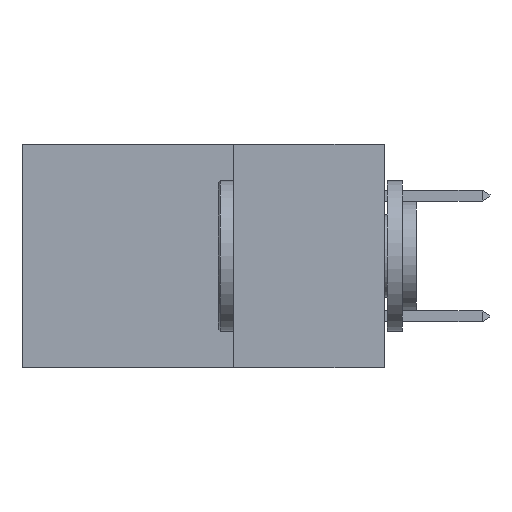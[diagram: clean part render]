
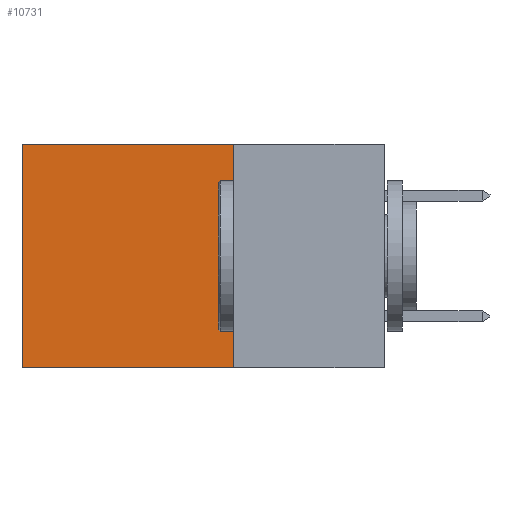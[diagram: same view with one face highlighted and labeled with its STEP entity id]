
A CAD part, left-side view. The second image highlights one B-rep face of the part: STEP entity #10731.
In plain terms, the highlighted planar face has unit normal (-1, 0, 0).
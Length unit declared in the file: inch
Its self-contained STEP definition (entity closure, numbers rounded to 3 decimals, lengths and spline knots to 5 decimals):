
#4 = DIRECTION ( 'NONE',  ( 0., 1., 0. ) ) ;
#1909 = VERTEX_POINT ( 'NONE', #10704 ) ;
#1969 = VECTOR ( 'NONE', #5695, 39.37008 ) ;
#2927 = ORIENTED_EDGE ( 'NONE', *, *, #12419, .T. ) ;
#3840 = VERTEX_POINT ( 'NONE', #6492 ) ;
#4129 = VECTOR ( 'NONE', #4, 39.37008 ) ;
#4249 = LINE ( 'NONE', #9013, #4129 ) ;
#4620 = VECTOR ( 'NONE', #12989, 39.37008 ) ;
#4773 = VERTEX_POINT ( 'NONE', #6629 ) ;
#5581 = CARTESIAN_POINT ( 'NONE',  ( 0.2875, 0.6, 0. ) ) ;
#5695 = DIRECTION ( 'NONE',  ( 0., 0., -1. ) ) ;
#6492 = CARTESIAN_POINT ( 'NONE',  ( 0.2875, 0.6, -0.37 ) ) ;
#6629 = CARTESIAN_POINT ( 'NONE',  ( 0.2875, 0.25, 0. ) ) ;
#7347 = ORIENTED_EDGE ( 'NONE', *, *, #15990, .F. ) ;
#7513 = ORIENTED_EDGE ( 'NONE', *, *, #19379, .T. ) ;
#8089 = CARTESIAN_POINT ( 'NONE',  ( 0.2875, 0.25, 0. ) ) ;
#8340 = DIRECTION ( 'NONE',  ( 1., 0., 0. ) ) ;
#9013 = CARTESIAN_POINT ( 'NONE',  ( 0.2875, 0.25, -0.37 ) ) ;
#10459 = CARTESIAN_POINT ( 'NONE',  ( 0.2875, 0.25, 0. ) ) ;
#10704 = CARTESIAN_POINT ( 'NONE',  ( 0.2875, 0.25, -0.37 ) ) ;
#10731 = ADVANCED_FACE ( 'NONE', ( #12785 ), #11434, .F. ) ;
#10888 = AXIS2_PLACEMENT_3D ( 'NONE', #16354, #8340, #11574 ) ;
#10932 = DIRECTION ( 'NONE',  ( 0., 0., -1. ) ) ;
#11126 = LINE ( 'NONE', #13688, #18423 ) ;
#11434 = PLANE ( 'NONE',  #10888 ) ;
#11574 = DIRECTION ( 'NONE',  ( 0., 0., -1. ) ) ;
#11868 = LINE ( 'NONE', #8089, #4620 ) ;
#11991 = VERTEX_POINT ( 'NONE', #5581 ) ;
#12419 = EDGE_CURVE ( 'NONE', #11991, #3840, #11126, .T. ) ;
#12785 = FACE_OUTER_BOUND ( 'NONE', #14713, .T. ) ;
#12989 = DIRECTION ( 'NONE',  ( 0., 1., 0. ) ) ;
#13688 = CARTESIAN_POINT ( 'NONE',  ( 0.2875, 0.6, 0. ) ) ;
#14713 = EDGE_LOOP ( 'NONE', ( #2927, #7347, #19468, #7513 ) ) ;
#15979 = LINE ( 'NONE', #10459, #1969 ) ;
#15990 = EDGE_CURVE ( 'NONE', #1909, #3840, #4249, .T. ) ;
#16309 = EDGE_CURVE ( 'NONE', #4773, #1909, #15979, .T. ) ;
#16354 = CARTESIAN_POINT ( 'NONE',  ( 0.2875, 0.25, 0. ) ) ;
#18423 = VECTOR ( 'NONE', #10932, 39.37008 ) ;
#19379 = EDGE_CURVE ( 'NONE', #4773, #11991, #11868, .T. ) ;
#19468 = ORIENTED_EDGE ( 'NONE', *, *, #16309, .F. ) ;
